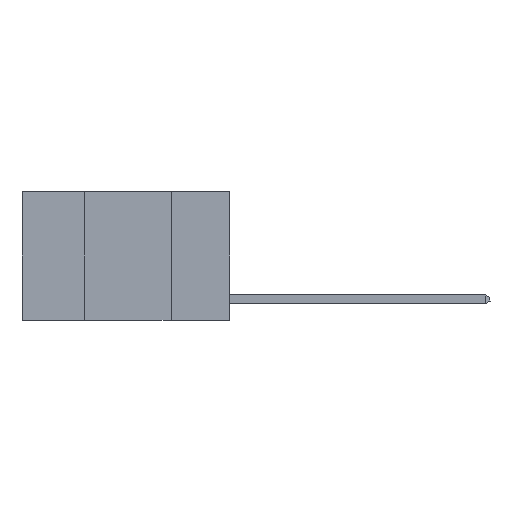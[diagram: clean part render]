
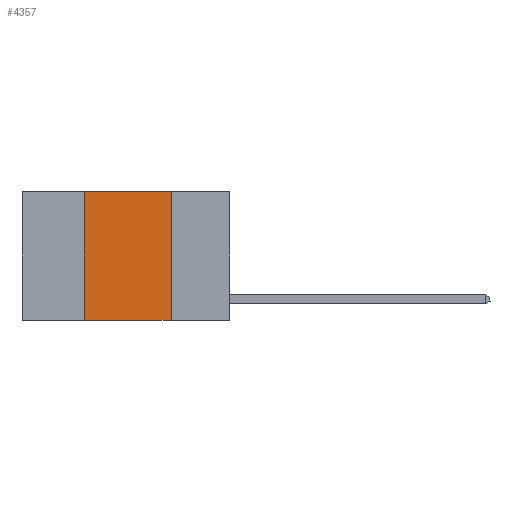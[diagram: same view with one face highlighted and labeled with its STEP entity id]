
A CAD part, left-side view. The second image highlights one B-rep face of the part: STEP entity #4357.
In plain terms, the highlighted planar face has unit normal (-1, 0, 0).
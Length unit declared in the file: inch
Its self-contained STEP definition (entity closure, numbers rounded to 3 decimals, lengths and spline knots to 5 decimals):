
#894 = PLANE ( 'NONE',  #6103 ) ;
#1014 = EDGE_CURVE ( 'NONE', #10429, #13316, #15257, .T. ) ;
#2139 = VECTOR ( 'NONE', #19209, 39.37008 ) ;
#2198 = ORIENTED_EDGE ( 'NONE', *, *, #1014, .F. ) ;
#2339 = EDGE_CURVE ( 'NONE', #10429, #8868, #19308, .T. ) ;
#3257 = CARTESIAN_POINT ( 'NONE',  ( 0., 0.42, 0. ) ) ;
#3340 = ORIENTED_EDGE ( 'NONE', *, *, #18183, .F. ) ;
#4357 = ADVANCED_FACE ( 'NONE', ( #5733 ), #894, .F. ) ;
#4473 = DIRECTION ( 'NONE',  ( 0., 0., -1. ) ) ;
#5289 = LINE ( 'NONE', #17090, #15444 ) ;
#5733 = FACE_OUTER_BOUND ( 'NONE', #10532, .T. ) ;
#5848 = DIRECTION ( 'NONE',  ( 0., 0., -1. ) ) ;
#6103 = AXIS2_PLACEMENT_3D ( 'NONE', #7355, #13398, #5848 ) ;
#7022 = CARTESIAN_POINT ( 'NONE',  ( 0., 0.6, -0.37 ) ) ;
#7126 = VECTOR ( 'NONE', #4473, 39.37008 ) ;
#7355 = CARTESIAN_POINT ( 'NONE',  ( 0., 0.6, 0. ) ) ;
#8868 = VERTEX_POINT ( 'NONE', #9843 ) ;
#9843 = CARTESIAN_POINT ( 'NONE',  ( 0., 0.17, -0.37 ) ) ;
#10429 = VERTEX_POINT ( 'NONE', #16925 ) ;
#10532 = EDGE_LOOP ( 'NONE', ( #13086, #3340, #2198, #16568 ) ) ;
#12354 = LINE ( 'NONE', #15352, #7126 ) ;
#12760 = DIRECTION ( 'NONE',  ( 0., -1., 0. ) ) ;
#13086 = ORIENTED_EDGE ( 'NONE', *, *, #13350, .F. ) ;
#13316 = VERTEX_POINT ( 'NONE', #3257 ) ;
#13350 = EDGE_CURVE ( 'NONE', #16314, #8868, #12354, .T. ) ;
#13398 = DIRECTION ( 'NONE',  ( 1., 0., 0. ) ) ;
#14405 = VECTOR ( 'NONE', #16654, 39.37008 ) ;
#15257 = LINE ( 'NONE', #16755, #14405 ) ;
#15352 = CARTESIAN_POINT ( 'NONE',  ( 0., 0.17, 0. ) ) ;
#15444 = VECTOR ( 'NONE', #12760, 39.37008 ) ;
#16314 = VERTEX_POINT ( 'NONE', #19195 ) ;
#16568 = ORIENTED_EDGE ( 'NONE', *, *, #2339, .T. ) ;
#16654 = DIRECTION ( 'NONE',  ( 0., 0., 1. ) ) ;
#16755 = CARTESIAN_POINT ( 'NONE',  ( 0., 0.42, 0. ) ) ;
#16925 = CARTESIAN_POINT ( 'NONE',  ( 0., 0.42, -0.37 ) ) ;
#17090 = CARTESIAN_POINT ( 'NONE',  ( 0., 0.6, 0. ) ) ;
#18183 = EDGE_CURVE ( 'NONE', #13316, #16314, #5289, .T. ) ;
#19195 = CARTESIAN_POINT ( 'NONE',  ( 0., 0.17, 0. ) ) ;
#19209 = DIRECTION ( 'NONE',  ( 0., -1., 0. ) ) ;
#19308 = LINE ( 'NONE', #7022, #2139 ) ;
